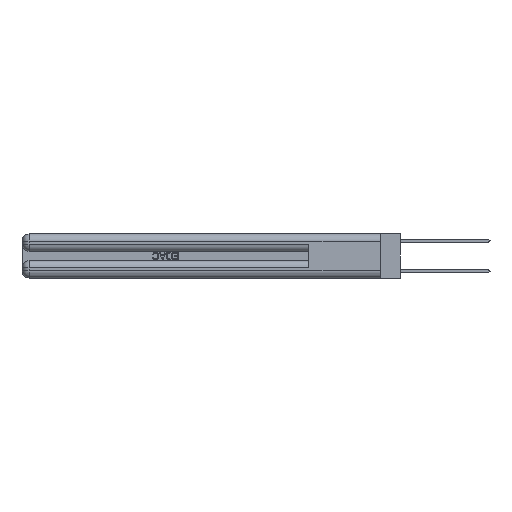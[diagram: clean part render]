
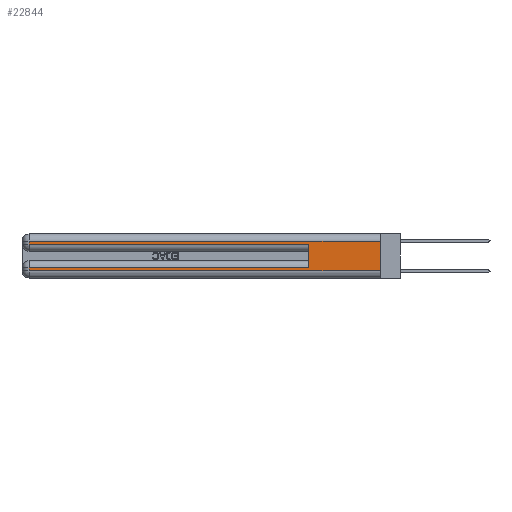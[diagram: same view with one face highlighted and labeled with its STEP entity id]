
A CAD part, left-side view. The second image highlights one B-rep face of the part: STEP entity #22844.
In plain terms, the highlighted planar face has unit normal (-1, 0, 0).
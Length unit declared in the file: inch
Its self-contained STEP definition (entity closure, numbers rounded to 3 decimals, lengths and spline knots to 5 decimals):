
#634 = CARTESIAN_POINT ( 'NONE',  ( 0., 0., 0.31 ) ) ;
#1124 = PLANE ( 'NONE',  #13744 ) ;
#1699 = CARTESIAN_POINT ( 'NONE',  ( 0., 0., 0.085 ) ) ;
#2178 = CARTESIAN_POINT ( 'NONE',  ( 0., 2.94, 0.285 ) ) ;
#2855 = CARTESIAN_POINT ( 'NONE',  ( 0., 0., 0.06 ) ) ;
#3562 = ORIENTED_EDGE ( 'NONE', *, *, #18716, .T. ) ;
#3972 = EDGE_CURVE ( 'NONE', #27949, #4262, #18351, .T. ) ;
#4262 = VERTEX_POINT ( 'NONE', #14589 ) ;
#4291 = CARTESIAN_POINT ( 'NONE',  ( 0., 0., 0.285 ) ) ;
#4496 = DIRECTION ( 'NONE',  ( 0., 1., 0. ) ) ;
#5752 = DIRECTION ( 'NONE',  ( 0., 0., -1. ) ) ;
#6982 = LINE ( 'NONE', #1699, #29507 ) ;
#7575 = ORIENTED_EDGE ( 'NONE', *, *, #8657, .T. ) ;
#7734 = VECTOR ( 'NONE', #5752, 39.37008 ) ;
#8108 = VECTOR ( 'NONE', #29105, 39.37008 ) ;
#8314 = CARTESIAN_POINT ( 'NONE',  ( 0., 0.6, 0.285 ) ) ;
#8537 = VECTOR ( 'NONE', #19611, 39.37008 ) ;
#8657 = EDGE_CURVE ( 'NONE', #4262, #13849, #26379, .T. ) ;
#8811 = DIRECTION ( 'NONE',  ( 1., 0., 0. ) ) ;
#9077 = LINE ( 'NONE', #32807, #14285 ) ;
#9675 = CARTESIAN_POINT ( 'NONE',  ( 0., 0., 0.06 ) ) ;
#11410 = CARTESIAN_POINT ( 'NONE',  ( 0., 2.94, 0.37 ) ) ;
#12242 = EDGE_CURVE ( 'NONE', #19721, #27949, #6982, .T. ) ;
#12518 = VERTEX_POINT ( 'NONE', #31881 ) ;
#12887 = EDGE_CURVE ( 'NONE', #33281, #13849, #9077, .T. ) ;
#13373 = EDGE_LOOP ( 'NONE', ( #18313, #19121, #24681, #3562, #25360, #15739, #26413, #7575 ) ) ;
#13744 = AXIS2_PLACEMENT_3D ( 'NONE', #19526, #8811, #29977 ) ;
#13849 = VERTEX_POINT ( 'NONE', #9675 ) ;
#14285 = VECTOR ( 'NONE', #27669, 39.37008 ) ;
#14589 = CARTESIAN_POINT ( 'NONE',  ( 0., 2.94, 0.06 ) ) ;
#15739 = ORIENTED_EDGE ( 'NONE', *, *, #12242, .T. ) ;
#15762 = CARTESIAN_POINT ( 'NONE',  ( 0., 0.6, 0.145 ) ) ;
#18313 = ORIENTED_EDGE ( 'NONE', *, *, #12887, .F. ) ;
#18351 = LINE ( 'NONE', #28631, #7734 ) ;
#18716 = EDGE_CURVE ( 'NONE', #20058, #21401, #24745, .T. ) ;
#19121 = ORIENTED_EDGE ( 'NONE', *, *, #23966, .T. ) ;
#19526 = CARTESIAN_POINT ( 'NONE',  ( 0., 0., 0.37 ) ) ;
#19611 = DIRECTION ( 'NONE',  ( 0., -1., 0. ) ) ;
#19721 = VERTEX_POINT ( 'NONE', #33215 ) ;
#19758 = DIRECTION ( 'NONE',  ( 0., 1., 0. ) ) ;
#20050 = VECTOR ( 'NONE', #26042, 39.37008 ) ;
#20058 = VERTEX_POINT ( 'NONE', #2178 ) ;
#20162 = LINE ( 'NONE', #27694, #32332 ) ;
#20971 = VECTOR ( 'NONE', #32246, 39.37008 ) ;
#21401 = VERTEX_POINT ( 'NONE', #8314 ) ;
#22844 = ADVANCED_FACE ( 'NONE', ( #29022 ), #1124, .F. ) ;
#22938 = LINE ( 'NONE', #15762, #8108 ) ;
#23966 = EDGE_CURVE ( 'NONE', #33281, #12518, #20162, .T. ) ;
#24033 = LINE ( 'NONE', #11410, #20971 ) ;
#24681 = ORIENTED_EDGE ( 'NONE', *, *, #25833, .T. ) ;
#24745 = LINE ( 'NONE', #4291, #8537 ) ;
#25360 = ORIENTED_EDGE ( 'NONE', *, *, #32270, .F. ) ;
#25833 = EDGE_CURVE ( 'NONE', #12518, #20058, #24033, .T. ) ;
#26042 = DIRECTION ( 'NONE',  ( 0., -1., 0. ) ) ;
#26379 = LINE ( 'NONE', #2855, #20050 ) ;
#26413 = ORIENTED_EDGE ( 'NONE', *, *, #3972, .T. ) ;
#27669 = DIRECTION ( 'NONE',  ( 0., 0., -1. ) ) ;
#27694 = CARTESIAN_POINT ( 'NONE',  ( 0., 0., 0.31 ) ) ;
#27949 = VERTEX_POINT ( 'NONE', #31200 ) ;
#28631 = CARTESIAN_POINT ( 'NONE',  ( 0., 2.94, 0.37 ) ) ;
#29022 = FACE_OUTER_BOUND ( 'NONE', #13373, .T. ) ;
#29105 = DIRECTION ( 'NONE',  ( 0., 0., 1. ) ) ;
#29507 = VECTOR ( 'NONE', #19758, 39.37008 ) ;
#29977 = DIRECTION ( 'NONE',  ( 0., 0., -1. ) ) ;
#31200 = CARTESIAN_POINT ( 'NONE',  ( 0., 2.94, 0.085 ) ) ;
#31881 = CARTESIAN_POINT ( 'NONE',  ( 0., 2.94, 0.31 ) ) ;
#32246 = DIRECTION ( 'NONE',  ( 0., 0., -1. ) ) ;
#32270 = EDGE_CURVE ( 'NONE', #19721, #21401, #22938, .T. ) ;
#32332 = VECTOR ( 'NONE', #4496, 39.37008 ) ;
#32807 = CARTESIAN_POINT ( 'NONE',  ( 0., 0., 0.37 ) ) ;
#33215 = CARTESIAN_POINT ( 'NONE',  ( 0., 0.6, 0.085 ) ) ;
#33281 = VERTEX_POINT ( 'NONE', #634 ) ;
